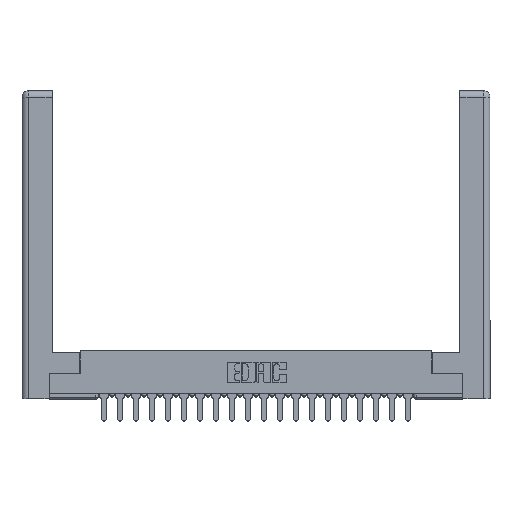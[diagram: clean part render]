
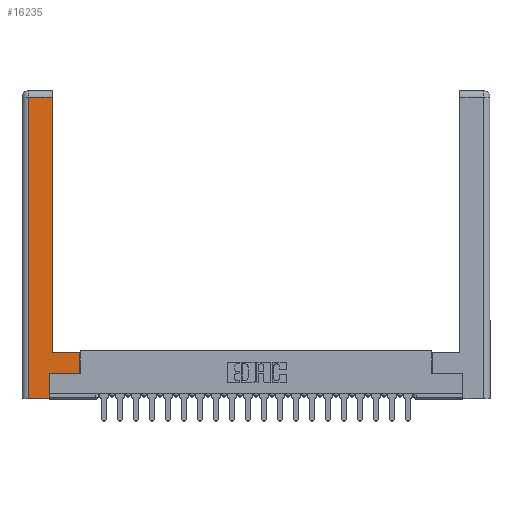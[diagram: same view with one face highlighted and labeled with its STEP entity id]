
A CAD part, top view. The second image highlights one B-rep face of the part: STEP entity #16235.
In plain terms, the highlighted planar face has unit normal (0, 0, 1).
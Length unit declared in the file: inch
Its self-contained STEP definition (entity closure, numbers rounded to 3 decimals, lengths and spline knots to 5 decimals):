
#101 = DIRECTION ( 'NONE',  ( 1., 0., 0. ) ) ;
#348 = LINE ( 'NONE', #5364, #11148 ) ;
#372 = EDGE_CURVE ( 'NONE', #5384, #737, #7668, .T. ) ;
#737 = VERTEX_POINT ( 'NONE', #6523 ) ;
#1349 = ORIENTED_EDGE ( 'NONE', *, *, #21261, .T. ) ;
#2096 = VECTOR ( 'NONE', #101, 39.37008 ) ;
#2643 = CARTESIAN_POINT ( 'NONE',  ( 0.0615, 2.94, 0. ) ) ;
#3185 = LINE ( 'NONE', #19105, #11813 ) ;
#3452 = ORIENTED_EDGE ( 'NONE', *, *, #17284, .T. ) ;
#3868 = LINE ( 'NONE', #3979, #12193 ) ;
#3979 = CARTESIAN_POINT ( 'NONE',  ( 0.0615, 0., 0. ) ) ;
#4025 = CARTESIAN_POINT ( 'NONE',  ( 0.565, 0.245, 0. ) ) ;
#4078 = CARTESIAN_POINT ( 'NONE',  ( 0.265, 0.245, 0. ) ) ;
#4243 = EDGE_CURVE ( 'NONE', #9237, #21942, #12461, .T. ) ;
#4309 = CARTESIAN_POINT ( 'NONE',  ( 0.295, 3., 0. ) ) ;
#5364 = CARTESIAN_POINT ( 'NONE',  ( 0.265, 0.245, 0. ) ) ;
#5384 = VERTEX_POINT ( 'NONE', #9642 ) ;
#5400 = VECTOR ( 'NONE', #5586, 39.37008 ) ;
#5586 = DIRECTION ( 'NONE',  ( -1., 0., 0. ) ) ;
#5605 = DIRECTION ( 'NONE',  ( 0., 1., 0. ) ) ;
#6523 = CARTESIAN_POINT ( 'NONE',  ( 0.295, 2.94, 0. ) ) ;
#6792 = DIRECTION ( 'NONE',  ( 1., 0., 0. ) ) ;
#7642 = LINE ( 'NONE', #2643, #20539 ) ;
#7668 = LINE ( 'NONE', #4309, #14246 ) ;
#8019 = CARTESIAN_POINT ( 'NONE',  ( 0., 0., 0. ) ) ;
#8556 = LINE ( 'NONE', #13590, #11059 ) ;
#8731 = ORIENTED_EDGE ( 'NONE', *, *, #17286, .T. ) ;
#9067 = CARTESIAN_POINT ( 'NONE',  ( 0.565, 0.45, 0. ) ) ;
#9237 = VERTEX_POINT ( 'NONE', #4078 ) ;
#9642 = CARTESIAN_POINT ( 'NONE',  ( 0.295, 0.45, 0. ) ) ;
#10233 = CARTESIAN_POINT ( 'NONE',  ( 0.0615, 0., 0. ) ) ;
#10824 = ORIENTED_EDGE ( 'NONE', *, *, #13189, .T. ) ;
#11059 = VECTOR ( 'NONE', #18984, 39.37008 ) ;
#11148 = VECTOR ( 'NONE', #5605, 39.37008 ) ;
#11201 = EDGE_LOOP ( 'NONE', ( #13273, #1349, #14277, #8731, #21896, #18152, #3452, #10824 ) ) ;
#11399 = DIRECTION ( 'NONE',  ( 0., 1., 0. ) ) ;
#11614 = DIRECTION ( 'NONE',  ( -1., 0., 0. ) ) ;
#11813 = VECTOR ( 'NONE', #6792, 39.37008 ) ;
#12193 = VECTOR ( 'NONE', #21290, 39.37008 ) ;
#12389 = CARTESIAN_POINT ( 'NONE',  ( 0.0615, 2.94, 0. ) ) ;
#12461 = LINE ( 'NONE', #14343, #2096 ) ;
#12594 = LINE ( 'NONE', #18015, #5400 ) ;
#13087 = PLANE ( 'NONE',  #20776 ) ;
#13189 = EDGE_CURVE ( 'NONE', #16574, #5384, #12594, .T. ) ;
#13273 = ORIENTED_EDGE ( 'NONE', *, *, #372, .T. ) ;
#13308 = DIRECTION ( 'NONE',  ( 0., 0., -1. ) ) ;
#13590 = CARTESIAN_POINT ( 'NONE',  ( 0.565, 0.45, 0. ) ) ;
#14246 = VECTOR ( 'NONE', #11399, 39.37008 ) ;
#14277 = ORIENTED_EDGE ( 'NONE', *, *, #17594, .T. ) ;
#14343 = CARTESIAN_POINT ( 'NONE',  ( 0.565, 0.245, 0. ) ) ;
#16235 = ADVANCED_FACE ( 'NONE', ( #18708 ), #13087, .F. ) ;
#16574 = VERTEX_POINT ( 'NONE', #9067 ) ;
#16891 = VERTEX_POINT ( 'NONE', #10233 ) ;
#17284 = EDGE_CURVE ( 'NONE', #21942, #16574, #8556, .T. ) ;
#17286 = EDGE_CURVE ( 'NONE', #16891, #20854, #3185, .T. ) ;
#17594 = EDGE_CURVE ( 'NONE', #20171, #16891, #3868, .T. ) ;
#18015 = CARTESIAN_POINT ( 'NONE',  ( 0.295, 0.45, 0. ) ) ;
#18152 = ORIENTED_EDGE ( 'NONE', *, *, #4243, .T. ) ;
#18471 = CARTESIAN_POINT ( 'NONE',  ( 0.265, 0., 0. ) ) ;
#18708 = FACE_OUTER_BOUND ( 'NONE', #11201, .T. ) ;
#18984 = DIRECTION ( 'NONE',  ( 0., 1., 0. ) ) ;
#19105 = CARTESIAN_POINT ( 'NONE',  ( 0.265, 0., 0. ) ) ;
#20171 = VERTEX_POINT ( 'NONE', #12389 ) ;
#20241 = DIRECTION ( 'NONE',  ( -1., 0., 0. ) ) ;
#20539 = VECTOR ( 'NONE', #11614, 39.37008 ) ;
#20776 = AXIS2_PLACEMENT_3D ( 'NONE', #8019, #13308, #20241 ) ;
#20854 = VERTEX_POINT ( 'NONE', #18471 ) ;
#21261 = EDGE_CURVE ( 'NONE', #737, #20171, #7642, .T. ) ;
#21290 = DIRECTION ( 'NONE',  ( 0., -1., 0. ) ) ;
#21896 = ORIENTED_EDGE ( 'NONE', *, *, #22272, .T. ) ;
#21942 = VERTEX_POINT ( 'NONE', #4025 ) ;
#22272 = EDGE_CURVE ( 'NONE', #20854, #9237, #348, .T. ) ;
